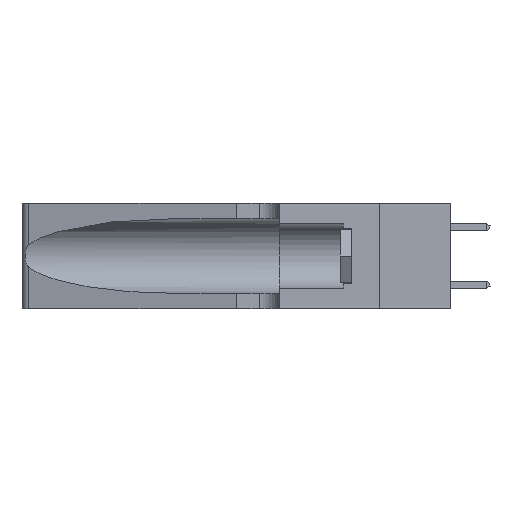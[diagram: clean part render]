
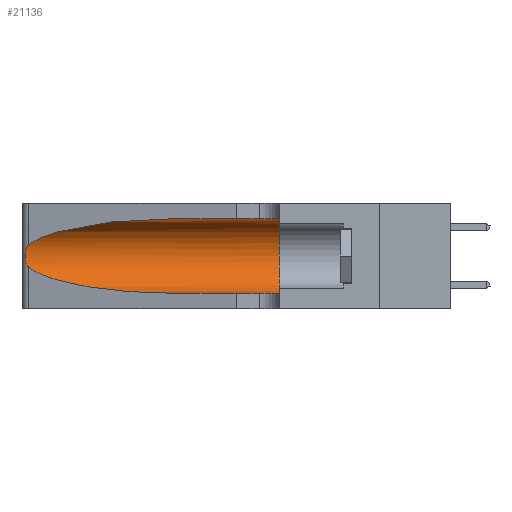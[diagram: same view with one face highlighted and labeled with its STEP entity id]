
A CAD part, left-side view. The second image highlights one B-rep face of the part: STEP entity #21136.
In plain terms, the highlighted cylindrical face has radius 3.308 mm (diameter 6.617 mm), a partial arc.
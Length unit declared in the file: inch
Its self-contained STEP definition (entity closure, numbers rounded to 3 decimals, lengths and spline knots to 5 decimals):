
#380 = CARTESIAN_POINT ( 'NONE',  ( 0.1305, 1.61858, 0.31525 ) ) ;
#602 = VERTEX_POINT ( 'NONE', #17010 ) ;
#606 = CARTESIAN_POINT ( 'NONE',  ( 0.1305, 0.72297, 0.31525 ) ) ;
#1543 = CARTESIAN_POINT ( 'NONE',  ( 0.25487, 1.22718, 0.14631 ) ) ;
#2050 = CARTESIAN_POINT ( 'NONE',  ( 0.18966, 0.96281, 0.31525 ) ) ;
#2198 = CARTESIAN_POINT ( 'NONE',  ( 0.2373, 1.15595, 0.28018 ) ) ;
#2428 = CARTESIAN_POINT ( 'NONE',  ( 0.1305, 0.72297, 0.05475 ) ) ;
#2591 = ORIENTED_EDGE ( 'NONE', *, *, #16275, .T. ) ;
#2939 = VERTEX_POINT ( 'NONE', #10564 ) ;
#2995 = VECTOR ( 'NONE', #4856, 39.37008 ) ;
#3039 = ORIENTED_EDGE ( 'NONE', *, *, #11583, .F. ) ;
#3214 = CARTESIAN_POINT ( 'NONE',  ( 0.25639, 1.23184, 0.21858 ) ) ;
#3477 = EDGE_LOOP ( 'NONE', ( #14104, #13569, #7338, #2591, #6871, #3039 ) ) ;
#3483 = CARTESIAN_POINT ( 'NONE',  ( 0.26075, 1.23896, 0.19203 ) ) ;
#4856 = DIRECTION ( 'NONE',  ( 0., -1., 0. ) ) ;
#4930 = DIRECTION ( 'NONE',  ( 0., 0., -1. ) ) ;
#5089 = FACE_OUTER_BOUND ( 'NONE', #3477, .T. ) ;
#5232 = VERTEX_POINT ( 'NONE', #7883 ) ;
#5233 = CARTESIAN_POINT ( 'NONE',  ( 0.25555, 1.22994, 0.2215 ) ) ;
#5275 = CARTESIAN_POINT ( 'NONE',  ( 0.26017, 1.23833, 0.17102 ) ) ;
#5830 = CIRCLE ( 'NONE', #12971, 0.13025 ) ;
#6447 = VECTOR ( 'NONE', #20504, 39.37008 ) ;
#6871 = ORIENTED_EDGE ( 'NONE', *, *, #13448, .F. ) ;
#7338 = ORIENTED_EDGE ( 'NONE', *, *, #14212, .T. ) ;
#7532 = CARTESIAN_POINT ( 'NONE',  ( 0.2373, 1.15595, 0.08982 ) ) ;
#7883 = CARTESIAN_POINT ( 'NONE',  ( 0.1305, 0.72297, 0.05475 ) ) ;
#8143 = CARTESIAN_POINT ( 'NONE',  ( 0.1305, 1.61858, 0.185 ) ) ;
#8316 = VERTEX_POINT ( 'NONE', #1543 ) ;
#9484 = CARTESIAN_POINT ( 'NONE',  ( 0.1305, 0.35, 0.31525 ) ) ;
#9567 = LINE ( 'NONE', #380, #6447 ) ;
#9575 =( BOUNDED_CURVE ( )  B_SPLINE_CURVE ( 3, ( #606, #2050, #2198, #13818 ),
 .UNSPECIFIED., .F., .F. ) 
 B_SPLINE_CURVE_WITH_KNOTS ( ( 4, 4 ),
 ( 1.5708, 2.84003 ),
 .UNSPECIFIED. ) 
 CURVE ( )  GEOMETRIC_REPRESENTATION_ITEM ( )  RATIONAL_B_SPLINE_CURVE ( ( 1., 0.87, 0.87, 1. ) ) 
 REPRESENTATION_ITEM ( '' )  );
#9597 = CARTESIAN_POINT ( 'NONE',  ( 0.25787, 1.23484, 0.2124 ) ) ;
#10152 = CARTESIAN_POINT ( 'NONE',  ( 0.25487, 1.22718, 0.14631 ) ) ;
#10505 = VERTEX_POINT ( 'NONE', #16541 ) ;
#10564 = CARTESIAN_POINT ( 'NONE',  ( 0.1305, 0.72297, 0.31525 ) ) ;
#11326 = CARTESIAN_POINT ( 'NONE',  ( 0.1305, 1.61858, 0.05475 ) ) ;
#11583 = EDGE_CURVE ( 'NONE', #2939, #15443, #9567, .T. ) ;
#11650 = EDGE_CURVE ( 'NONE', #2939, #10505, #9575, .T. ) ;
#12360 = CARTESIAN_POINT ( 'NONE',  ( 0.25487, 1.22718, 0.14631 ) ) ;
#12971 = AXIS2_PLACEMENT_3D ( 'NONE', #20226, #15508, #20294 ) ;
#13143 = CARTESIAN_POINT ( 'NONE',  ( 0.25854, 1.2359, 0.20912 ) ) ;
#13448 = EDGE_CURVE ( 'NONE', #15443, #602, #5830, .T. ) ;
#13511 = CARTESIAN_POINT ( 'NONE',  ( 0.25487, 1.22718, 0.22369 ) ) ;
#13569 = ORIENTED_EDGE ( 'NONE', *, *, #15381, .T. ) ;
#13818 = CARTESIAN_POINT ( 'NONE',  ( 0.25487, 1.22718, 0.22369 ) ) ;
#14104 = ORIENTED_EDGE ( 'NONE', *, *, #11650, .T. ) ;
#14212 = EDGE_CURVE ( 'NONE', #8316, #5232, #14771, .T. ) ;
#14771 =( BOUNDED_CURVE ( )  B_SPLINE_CURVE ( 3, ( #12360, #7532, #17166, #2428 ),
 .UNSPECIFIED., .F., .F. ) 
 B_SPLINE_CURVE_WITH_KNOTS ( ( 4, 4 ),
 ( 3.44316, 4.71239 ),
 .UNSPECIFIED. ) 
 CURVE ( )  GEOMETRIC_REPRESENTATION_ITEM ( )  RATIONAL_B_SPLINE_CURVE ( ( 1., 0.87, 0.87, 1. ) ) 
 REPRESENTATION_ITEM ( '' )  );
#15262 = CARTESIAN_POINT ( 'NONE',  ( 0.26075, 1.23896, 0.178 ) ) ;
#15381 = EDGE_CURVE ( 'NONE', #10505, #8316, #20218, .T. ) ;
#15443 = VERTEX_POINT ( 'NONE', #9484 ) ;
#15508 = DIRECTION ( 'NONE',  ( 0., 1., 0. ) ) ;
#16275 = EDGE_CURVE ( 'NONE', #5232, #602, #16999, .T. ) ;
#16541 = CARTESIAN_POINT ( 'NONE',  ( 0.25487, 1.22718, 0.22369 ) ) ;
#16638 = CARTESIAN_POINT ( 'NONE',  ( 0.26018, 1.23835, 0.19895 ) ) ;
#16708 = CARTESIAN_POINT ( 'NONE',  ( 0.25856, 1.23593, 0.16098 ) ) ;
#16999 = LINE ( 'NONE', #11326, #2995 ) ;
#17010 = CARTESIAN_POINT ( 'NONE',  ( 0.1305, 0.35, 0.05475 ) ) ;
#17166 = CARTESIAN_POINT ( 'NONE',  ( 0.18966, 0.96281, 0.05475 ) ) ;
#18218 = DIRECTION ( 'NONE',  ( 0., -1., 0. ) ) ;
#18225 = CARTESIAN_POINT ( 'NONE',  ( 0.25639, 1.23186, 0.15144 ) ) ;
#18289 = CARTESIAN_POINT ( 'NONE',  ( 0.25555, 1.22993, 0.14849 ) ) ;
#19755 = AXIS2_PLACEMENT_3D ( 'NONE', #8143, #18218, #4930 ) ;
#20109 = CARTESIAN_POINT ( 'NONE',  ( 0.25789, 1.23486, 0.15765 ) ) ;
#20218 = B_SPLINE_CURVE_WITH_KNOTS ( 'NONE', 3,
 ( #13511, #5233, #3214, #9597, #13143, #16638, #3483, #15262, #5275, #16708, #20109, #18225, #18289, #10152 ),
 .UNSPECIFIED., .F., .F.,
 ( 4, 2, 2, 2, 2, 2, 4 ),
 ( 0., 0.00027, 0.00053, 0.00107, 0.0016, 0.00187, 0.00214 ),
 .UNSPECIFIED. ) ;
#20226 = CARTESIAN_POINT ( 'NONE',  ( 0.1305, 0.35, 0.185 ) ) ;
#20294 = DIRECTION ( 'NONE',  ( 0., 0., 1. ) ) ;
#20504 = DIRECTION ( 'NONE',  ( 0., -1., 0. ) ) ;
#21136 = ADVANCED_FACE ( 'NONE', ( #5089 ), #21209, .F. ) ;
#21209 = CYLINDRICAL_SURFACE ( 'NONE', #19755, 0.13025 ) ;
